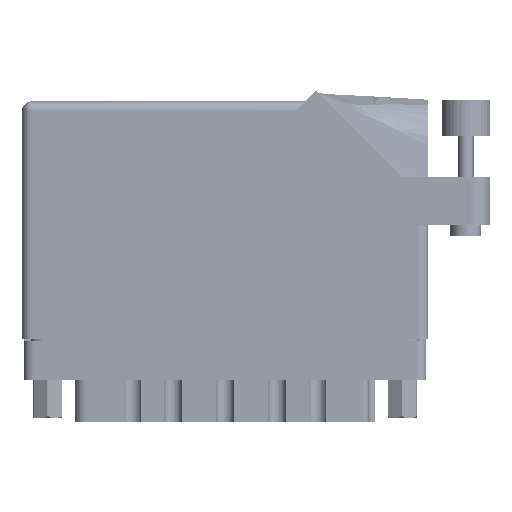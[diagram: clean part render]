
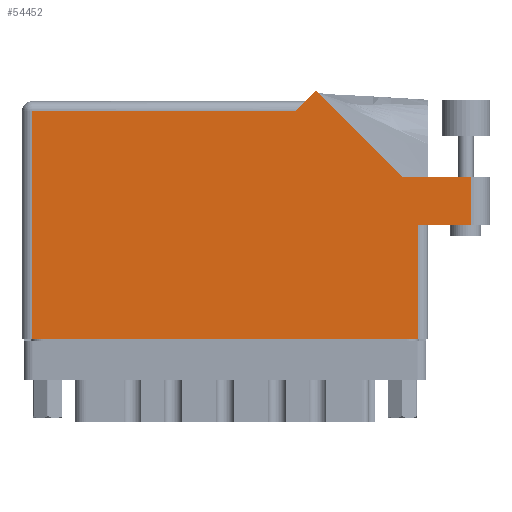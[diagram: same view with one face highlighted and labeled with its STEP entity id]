
A CAD part, front view. The second image highlights one B-rep face of the part: STEP entity #54452.
In plain terms, the highlighted face is planar.
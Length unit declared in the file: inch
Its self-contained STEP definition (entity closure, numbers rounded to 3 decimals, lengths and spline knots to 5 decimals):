
#547 = CARTESIAN_POINT ( 'NONE',  ( 0.062, 0., 0. ) ) ;
#3145 = EDGE_CURVE ( 'NONE', #14064, #31632, #15664, .T. ) ;
#4733 = CARTESIAN_POINT ( 'NONE',  ( 1.757, 1.468, 0. ) ) ;
#6563 = DIRECTION ( 'NONE',  ( -0.707, 0.707, 0. ) ) ;
#6893 = VECTOR ( 'NONE', #32927, 39.37008 ) ;
#6980 = PLANE ( 'NONE',  #37295 ) ;
#7391 = LINE ( 'NONE', #53123, #59376 ) ;
#7639 = CARTESIAN_POINT ( 'NONE',  ( 2.55, 0.737, 0. ) ) ;
#9351 = ORIENTED_EDGE ( 'NONE', *, *, #11107, .T. ) ;
#9623 = VECTOR ( 'NONE', #28229, 39.37008 ) ;
#11107 = EDGE_CURVE ( 'NONE', #55675, #26545, #7391, .T. ) ;
#11283 = CARTESIAN_POINT ( 'NONE',  ( 0., 1.468, 0. ) ) ;
#11597 = VERTEX_POINT ( 'NONE', #57773 ) ;
#11928 = VECTOR ( 'NONE', #52103, 39.37008 ) ;
#13245 = CARTESIAN_POINT ( 'NONE',  ( 1.88971, 1.60071, 0. ) ) ;
#13949 = CARTESIAN_POINT ( 'NONE',  ( 2.44642, 1.044, 0. ) ) ;
#14064 = VERTEX_POINT ( 'NONE', #7639 ) ;
#15041 = ORIENTED_EDGE ( 'NONE', *, *, #3145, .T. ) ;
#15628 = DIRECTION ( 'NONE',  ( 0., 0., -1. ) ) ;
#15664 = LINE ( 'NONE', #33843, #29140 ) ;
#18353 = CARTESIAN_POINT ( 'NONE',  ( 3.012, 1.044, 0. ) ) ;
#18797 = CARTESIAN_POINT ( 'NONE',  ( 2.887, 1.044, 0. ) ) ;
#18940 = DIRECTION ( 'NONE',  ( 1., 0., 0. ) ) ;
#23255 = VERTEX_POINT ( 'NONE', #13949 ) ;
#25667 = CARTESIAN_POINT ( 'NONE',  ( 0., 1.53, 0. ) ) ;
#26545 = VERTEX_POINT ( 'NONE', #42191 ) ;
#27051 = VECTOR ( 'NONE', #6563, 39.37008 ) ;
#28022 = FACE_OUTER_BOUND ( 'NONE', #45303, .T. ) ;
#28229 = DIRECTION ( 'NONE',  ( 0., 1., 0. ) ) ;
#29140 = VECTOR ( 'NONE', #18940, 39.37008 ) ;
#30109 = ORIENTED_EDGE ( 'NONE', *, *, #47126, .T. ) ;
#30163 = EDGE_CURVE ( 'NONE', #26545, #14064, #52209, .T. ) ;
#30517 = EDGE_CURVE ( 'NONE', #11597, #55675, #48377, .T. ) ;
#31232 = DIRECTION ( 'NONE',  ( 0., 1., 0. ) ) ;
#31632 = VERTEX_POINT ( 'NONE', #62042 ) ;
#31859 = VECTOR ( 'NONE', #32559, 39.37008 ) ;
#32559 = DIRECTION ( 'NONE',  ( -0.707, -0.707, 0. ) ) ;
#32664 = LINE ( 'NONE', #61486, #31859 ) ;
#32927 = DIRECTION ( 'NONE',  ( 0., -1., 0. ) ) ;
#33843 = CARTESIAN_POINT ( 'NONE',  ( 2.612, 0.737, 0. ) ) ;
#33887 = DIRECTION ( 'NONE',  ( 1., 0., 0. ) ) ;
#37295 = AXIS2_PLACEMENT_3D ( 'NONE', #25667, #15628, #50154 ) ;
#37523 = LINE ( 'NONE', #18353, #11928 ) ;
#38331 = ORIENTED_EDGE ( 'NONE', *, *, #56256, .T. ) ;
#38660 = VECTOR ( 'NONE', #45404, 39.37008 ) ;
#38773 = VERTEX_POINT ( 'NONE', #13245 ) ;
#38871 = EDGE_CURVE ( 'NONE', #38773, #62130, #32664, .T. ) ;
#39231 = EDGE_CURVE ( 'NONE', #62130, #11597, #53774, .T. ) ;
#39310 = VECTOR ( 'NONE', #31232, 39.37008 ) ;
#40341 = CARTESIAN_POINT ( 'NONE',  ( 2.55, 0.737, 0. ) ) ;
#42191 = CARTESIAN_POINT ( 'NONE',  ( 2.55, 0., 0. ) ) ;
#43533 = ORIENTED_EDGE ( 'NONE', *, *, #30517, .T. ) ;
#43735 = ORIENTED_EDGE ( 'NONE', *, *, #38871, .T. ) ;
#44130 = EDGE_CURVE ( 'NONE', #31632, #49482, #48081, .T. ) ;
#45110 = CARTESIAN_POINT ( 'NONE',  ( 2.44642, 1.044, 0. ) ) ;
#45303 = EDGE_LOOP ( 'NONE', ( #15041, #52063, #30109, #38331, #43735, #53586, #43533, #9351, #60281 ) ) ;
#45404 = DIRECTION ( 'NONE',  ( -1., 0., 0. ) ) ;
#47126 = EDGE_CURVE ( 'NONE', #49482, #23255, #37523, .T. ) ;
#48081 = LINE ( 'NONE', #18797, #9623 ) ;
#48377 = LINE ( 'NONE', #56786, #6893 ) ;
#49470 = CARTESIAN_POINT ( 'NONE',  ( 2.887, 1.044, 0. ) ) ;
#49482 = VERTEX_POINT ( 'NONE', #49470 ) ;
#49706 = LINE ( 'NONE', #45110, #27051 ) ;
#50154 = DIRECTION ( 'NONE',  ( -1., 0., 0. ) ) ;
#52063 = ORIENTED_EDGE ( 'NONE', *, *, #44130, .T. ) ;
#52103 = DIRECTION ( 'NONE',  ( -1., 0., 0. ) ) ;
#52209 = LINE ( 'NONE', #40341, #39310 ) ;
#53123 = CARTESIAN_POINT ( 'NONE',  ( 0., 0., 0. ) ) ;
#53586 = ORIENTED_EDGE ( 'NONE', *, *, #39231, .T. ) ;
#53774 = LINE ( 'NONE', #11283, #38660 ) ;
#54452 = ADVANCED_FACE ( 'NONE', ( #28022 ), #6980, .F. ) ;
#55675 = VERTEX_POINT ( 'NONE', #547 ) ;
#56256 = EDGE_CURVE ( 'NONE', #23255, #38773, #49706, .T. ) ;
#56786 = CARTESIAN_POINT ( 'NONE',  ( 0.062, 0., 0. ) ) ;
#57773 = CARTESIAN_POINT ( 'NONE',  ( 0.062, 1.468, 0. ) ) ;
#59376 = VECTOR ( 'NONE', #33887, 39.37008 ) ;
#60281 = ORIENTED_EDGE ( 'NONE', *, *, #30163, .T. ) ;
#61486 = CARTESIAN_POINT ( 'NONE',  ( 1.819, 1.53, 0. ) ) ;
#62042 = CARTESIAN_POINT ( 'NONE',  ( 2.887, 0.737, 0. ) ) ;
#62130 = VERTEX_POINT ( 'NONE', #4733 ) ;
